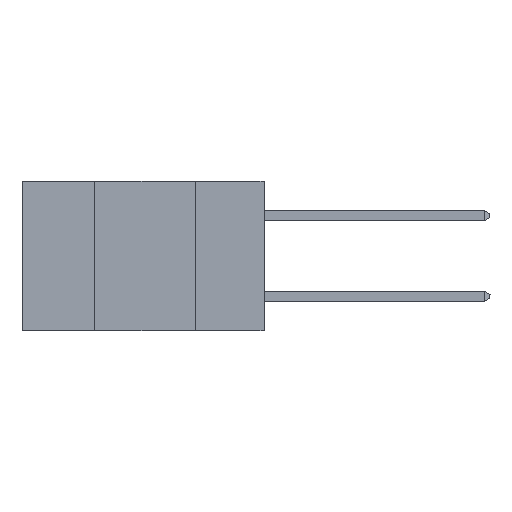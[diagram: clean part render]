
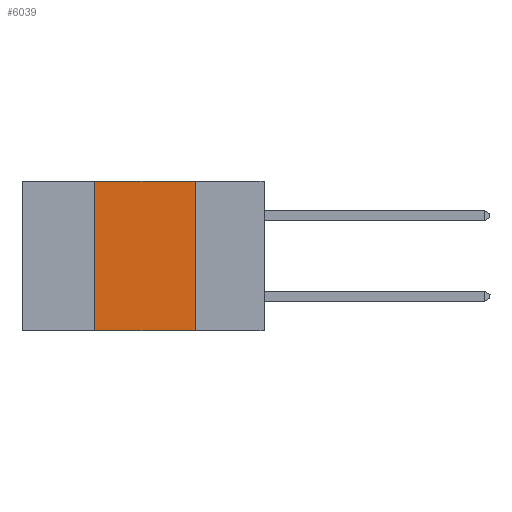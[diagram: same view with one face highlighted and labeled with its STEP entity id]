
A CAD part, left-side view. The second image highlights one B-rep face of the part: STEP entity #6039.
In plain terms, the highlighted planar face has unit normal (-1, 0, 0).
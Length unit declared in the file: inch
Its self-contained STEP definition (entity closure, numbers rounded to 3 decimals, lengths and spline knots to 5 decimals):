
#2918 = VERTEX_POINT ( 'NONE', #12290 ) ;
#3307 = CARTESIAN_POINT ( 'NONE',  ( 0., 0.6, -0.37 ) ) ;
#3431 = DIRECTION ( 'NONE',  ( 0., 0., -1. ) ) ;
#3519 = DIRECTION ( 'NONE',  ( 1., 0., 0. ) ) ;
#5008 = AXIS2_PLACEMENT_3D ( 'NONE', #18682, #3519, #3431 ) ;
#5264 = DIRECTION ( 'NONE',  ( 0., -1., 0. ) ) ;
#5514 = LINE ( 'NONE', #10951, #22098 ) ;
#6039 = ADVANCED_FACE ( 'NONE', ( #18840 ), #22493, .F. ) ;
#6322 = ORIENTED_EDGE ( 'NONE', *, *, #13015, .F. ) ;
#6550 = EDGE_CURVE ( 'NONE', #13558, #20611, #18812, .T. ) ;
#8715 = DIRECTION ( 'NONE',  ( 0., 0., 1. ) ) ;
#8895 = VECTOR ( 'NONE', #14815, 39.37008 ) ;
#9251 = VECTOR ( 'NONE', #5264, 39.37008 ) ;
#9406 = CARTESIAN_POINT ( 'NONE',  ( 0., 0.6, 0. ) ) ;
#10224 = CARTESIAN_POINT ( 'NONE',  ( 0., 0.17, -0.37 ) ) ;
#10951 = CARTESIAN_POINT ( 'NONE',  ( 0., 0.17, 0. ) ) ;
#12290 = CARTESIAN_POINT ( 'NONE',  ( 0., 0.17, 0. ) ) ;
#12427 = CARTESIAN_POINT ( 'NONE',  ( 0., 0.42, 0. ) ) ;
#13015 = EDGE_CURVE ( 'NONE', #20611, #2918, #15092, .T. ) ;
#13558 = VERTEX_POINT ( 'NONE', #20438 ) ;
#14501 = EDGE_LOOP ( 'NONE', ( #23066, #6322, #22530, #17342 ) ) ;
#14815 = DIRECTION ( 'NONE',  ( 0., -1., 0. ) ) ;
#14900 = EDGE_CURVE ( 'NONE', #2918, #15557, #5514, .T. ) ;
#15092 = LINE ( 'NONE', #9406, #8895 ) ;
#15557 = VERTEX_POINT ( 'NONE', #10224 ) ;
#17342 = ORIENTED_EDGE ( 'NONE', *, *, #24292, .T. ) ;
#18682 = CARTESIAN_POINT ( 'NONE',  ( 0., 0.6, 0. ) ) ;
#18812 = LINE ( 'NONE', #22299, #20021 ) ;
#18840 = FACE_OUTER_BOUND ( 'NONE', #14501, .T. ) ;
#20021 = VECTOR ( 'NONE', #8715, 39.37008 ) ;
#20438 = CARTESIAN_POINT ( 'NONE',  ( 0., 0.42, -0.37 ) ) ;
#20611 = VERTEX_POINT ( 'NONE', #12427 ) ;
#21004 = LINE ( 'NONE', #3307, #9251 ) ;
#22098 = VECTOR ( 'NONE', #22734, 39.37008 ) ;
#22299 = CARTESIAN_POINT ( 'NONE',  ( 0., 0.42, 0. ) ) ;
#22493 = PLANE ( 'NONE',  #5008 ) ;
#22530 = ORIENTED_EDGE ( 'NONE', *, *, #6550, .F. ) ;
#22734 = DIRECTION ( 'NONE',  ( 0., 0., -1. ) ) ;
#23066 = ORIENTED_EDGE ( 'NONE', *, *, #14900, .F. ) ;
#24292 = EDGE_CURVE ( 'NONE', #13558, #15557, #21004, .T. ) ;
